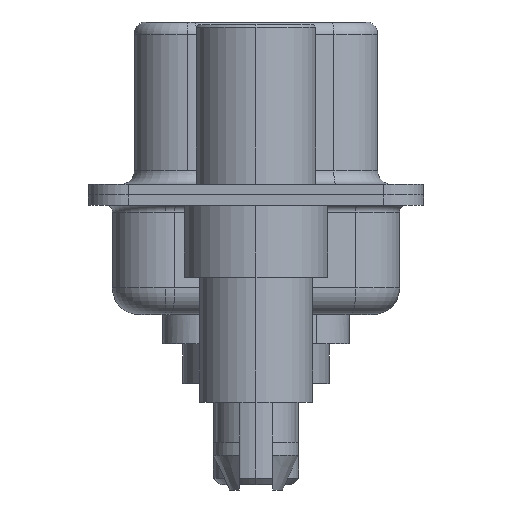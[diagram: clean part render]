
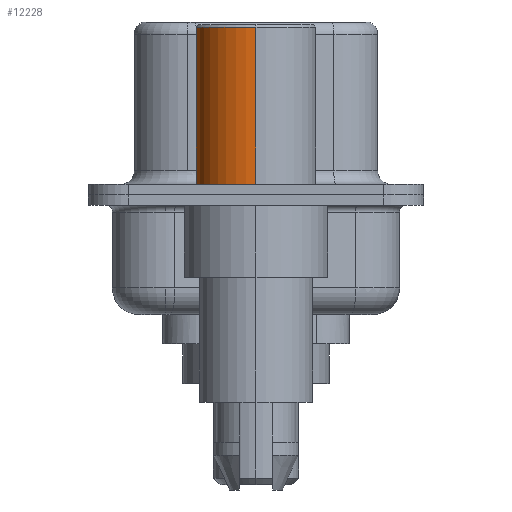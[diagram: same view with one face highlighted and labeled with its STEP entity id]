
A CAD part, left-side view. The second image highlights one B-rep face of the part: STEP entity #12228.
In plain terms, the highlighted cylindrical face has radius 2.25 mm (diameter 4.5 mm), a partial arc.
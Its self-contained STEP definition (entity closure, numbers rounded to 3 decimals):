
#209 = EDGE_CURVE ( 'NONE', #6195, #14672, #6445, .T. ) ;
#495 = AXIS2_PLACEMENT_3D ( 'NONE', #3363, #15653, #10612 ) ;
#836 = ORIENTED_EDGE ( 'NONE', *, *, #852, .T. ) ;
#852 = EDGE_CURVE ( 'NONE', #13824, #14672, #868, .T. ) ;
#868 = LINE ( 'NONE', #11694, #4119 ) ;
#951 = AXIS2_PLACEMENT_3D ( 'NONE', #991, #9438, #2195 ) ;
#991 = CARTESIAN_POINT ( 'NONE',  ( 0., 0., 0.4 ) ) ;
#1301 = ORIENTED_EDGE ( 'NONE', *, *, #209, .F. ) ;
#2109 = AXIS2_PLACEMENT_3D ( 'NONE', #4278, #8985, #14359 ) ;
#2195 = DIRECTION ( 'NONE',  ( 1., 0., 0. ) ) ;
#3363 = CARTESIAN_POINT ( 'NONE',  ( 0., 0., 0.581 ) ) ;
#3596 = EDGE_CURVE ( 'NONE', #14524, #6195, #14788, .T. ) ;
#4119 = VECTOR ( 'NONE', #11801, 1000. ) ;
#4278 = CARTESIAN_POINT ( 'NONE',  ( 0., 0., 6.3 ) ) ;
#4308 = CYLINDRICAL_SURFACE ( 'NONE', #495, 2.25 ) ;
#5434 = CARTESIAN_POINT ( 'NONE',  ( 2.25, 0., 0.4 ) ) ;
#6192 = DIRECTION ( 'NONE',  ( 0., 0., 1. ) ) ;
#6195 = VERTEX_POINT ( 'NONE', #8538 ) ;
#6445 = CIRCLE ( 'NONE', #2109, 2.25 ) ;
#6810 = CIRCLE ( 'NONE', #951, 2.25 ) ;
#6953 = CARTESIAN_POINT ( 'NONE',  ( -2.25, 0., 6.3 ) ) ;
#7223 = ORIENTED_EDGE ( 'NONE', *, *, #3596, .F. ) ;
#7453 = VECTOR ( 'NONE', #6192, 1000. ) ;
#8515 = CARTESIAN_POINT ( 'NONE',  ( 2.25, 0., 0.581 ) ) ;
#8538 = CARTESIAN_POINT ( 'NONE',  ( 2.25, 0., 6.3 ) ) ;
#8985 = DIRECTION ( 'NONE',  ( 0., 0., 1. ) ) ;
#9438 = DIRECTION ( 'NONE',  ( 0., 0., 1. ) ) ;
#10612 = DIRECTION ( 'NONE',  ( 1., 0., 0. ) ) ;
#11073 = EDGE_LOOP ( 'NONE', ( #12936, #836, #1301, #7223 ) ) ;
#11171 = CARTESIAN_POINT ( 'NONE',  ( -2.25, 0., 0.4 ) ) ;
#11526 = FACE_OUTER_BOUND ( 'NONE', #11073, .T. ) ;
#11694 = CARTESIAN_POINT ( 'NONE',  ( -2.25, 0., 0.581 ) ) ;
#11801 = DIRECTION ( 'NONE',  ( 0., 0., 1. ) ) ;
#12228 = ADVANCED_FACE ( 'NONE', ( #11526 ), #4308, .T. ) ;
#12936 = ORIENTED_EDGE ( 'NONE', *, *, #15791, .T. ) ;
#13824 = VERTEX_POINT ( 'NONE', #11171 ) ;
#14359 = DIRECTION ( 'NONE',  ( 1., 0., 0. ) ) ;
#14524 = VERTEX_POINT ( 'NONE', #5434 ) ;
#14672 = VERTEX_POINT ( 'NONE', #6953 ) ;
#14788 = LINE ( 'NONE', #8515, #7453 ) ;
#15653 = DIRECTION ( 'NONE',  ( 0., 0., 1. ) ) ;
#15791 = EDGE_CURVE ( 'NONE', #14524, #13824, #6810, .T. ) ;
